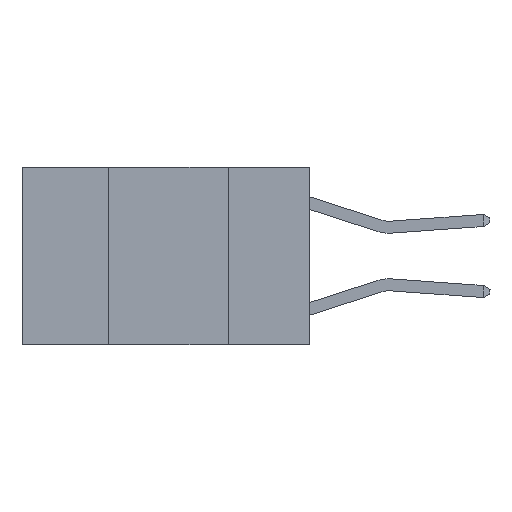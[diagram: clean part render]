
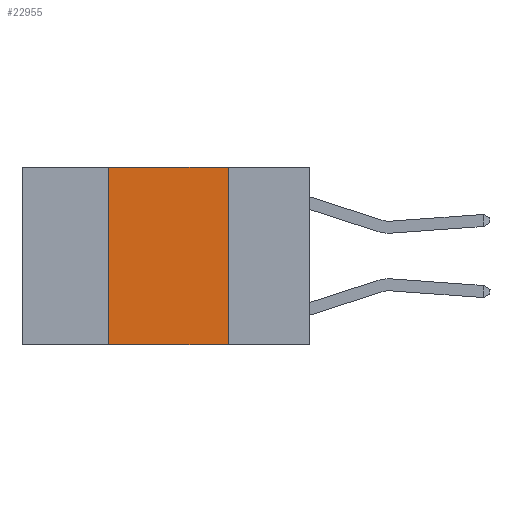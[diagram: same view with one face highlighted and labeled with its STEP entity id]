
A CAD part, left-side view. The second image highlights one B-rep face of the part: STEP entity #22955.
In plain terms, the highlighted planar face has unit normal (-1, 0, 0).
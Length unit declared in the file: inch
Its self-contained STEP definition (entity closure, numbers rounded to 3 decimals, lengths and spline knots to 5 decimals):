
#515 = DIRECTION ( 'NONE',  ( 0., -1., 0. ) ) ;
#1158 = EDGE_CURVE ( 'NONE', #12453, #2939, #9403, .T. ) ;
#2159 = CARTESIAN_POINT ( 'NONE',  ( 0., 0.42, -0.37 ) ) ;
#2354 = ORIENTED_EDGE ( 'NONE', *, *, #9119, .T. ) ;
#2423 = LINE ( 'NONE', #16863, #21875 ) ;
#2939 = VERTEX_POINT ( 'NONE', #20624 ) ;
#3689 = AXIS2_PLACEMENT_3D ( 'NONE', #15498, #6368, #19187 ) ;
#4508 = ORIENTED_EDGE ( 'NONE', *, *, #20597, .F. ) ;
#4528 = VECTOR ( 'NONE', #23240, 39.37008 ) ;
#4837 = EDGE_CURVE ( 'NONE', #11537, #12453, #2423, .T. ) ;
#5884 = DIRECTION ( 'NONE',  ( 0., -1., 0. ) ) ;
#6368 = DIRECTION ( 'NONE',  ( 1., 0., 0. ) ) ;
#6859 = CARTESIAN_POINT ( 'NONE',  ( 0., 0.17, 0. ) ) ;
#9119 = EDGE_CURVE ( 'NONE', #17877, #2939, #14576, .T. ) ;
#9403 = LINE ( 'NONE', #6859, #4528 ) ;
#9450 = LINE ( 'NONE', #9878, #23435 ) ;
#9878 = CARTESIAN_POINT ( 'NONE',  ( 0., 0.42, 0. ) ) ;
#11346 = ORIENTED_EDGE ( 'NONE', *, *, #1158, .F. ) ;
#11449 = CARTESIAN_POINT ( 'NONE',  ( 0., 0.17, 0. ) ) ;
#11537 = VERTEX_POINT ( 'NONE', #23198 ) ;
#12453 = VERTEX_POINT ( 'NONE', #11449 ) ;
#13863 = EDGE_LOOP ( 'NONE', ( #11346, #15301, #4508, #2354 ) ) ;
#14576 = LINE ( 'NONE', #22407, #18861 ) ;
#15301 = ORIENTED_EDGE ( 'NONE', *, *, #4837, .F. ) ;
#15498 = CARTESIAN_POINT ( 'NONE',  ( 0., 0.6, 0. ) ) ;
#15970 = FACE_OUTER_BOUND ( 'NONE', #13863, .T. ) ;
#16863 = CARTESIAN_POINT ( 'NONE',  ( 0., 0.6, 0. ) ) ;
#17368 = PLANE ( 'NONE',  #3689 ) ;
#17877 = VERTEX_POINT ( 'NONE', #2159 ) ;
#18861 = VECTOR ( 'NONE', #515, 39.37008 ) ;
#19187 = DIRECTION ( 'NONE',  ( 0., 0., -1. ) ) ;
#20597 = EDGE_CURVE ( 'NONE', #17877, #11537, #9450, .T. ) ;
#20624 = CARTESIAN_POINT ( 'NONE',  ( 0., 0.17, -0.37 ) ) ;
#21875 = VECTOR ( 'NONE', #5884, 39.37008 ) ;
#22407 = CARTESIAN_POINT ( 'NONE',  ( 0., 0.6, -0.37 ) ) ;
#22639 = DIRECTION ( 'NONE',  ( 0., 0., 1. ) ) ;
#22955 = ADVANCED_FACE ( 'NONE', ( #15970 ), #17368, .F. ) ;
#23198 = CARTESIAN_POINT ( 'NONE',  ( 0., 0.42, 0. ) ) ;
#23240 = DIRECTION ( 'NONE',  ( 0., 0., -1. ) ) ;
#23435 = VECTOR ( 'NONE', #22639, 39.37008 ) ;
